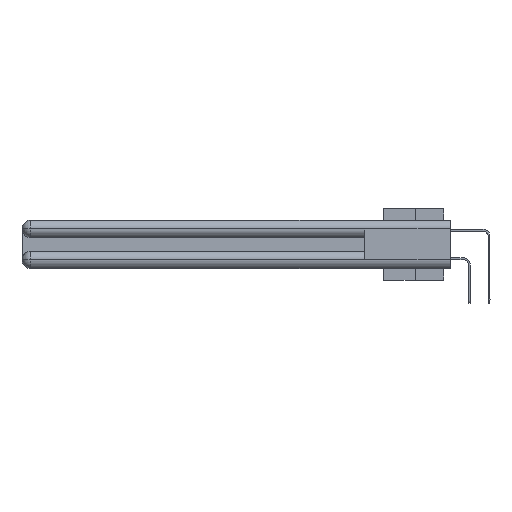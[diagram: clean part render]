
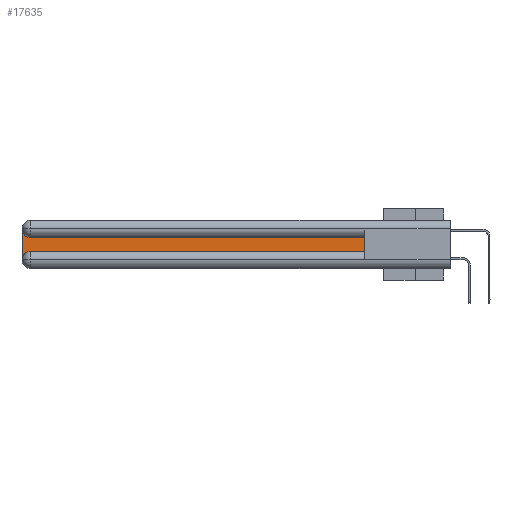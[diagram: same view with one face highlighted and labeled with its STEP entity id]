
A CAD part, left-side view. The second image highlights one B-rep face of the part: STEP entity #17635.
In plain terms, the highlighted planar face has unit normal (-1, 0, 0).
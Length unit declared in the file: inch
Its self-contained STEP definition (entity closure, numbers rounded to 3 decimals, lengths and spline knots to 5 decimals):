
#868 = VERTEX_POINT ( 'NONE', #5775 ) ;
#2789 = VECTOR ( 'NONE', #22124, 39.37008 ) ;
#3018 = VERTEX_POINT ( 'NONE', #8753 ) ;
#3198 = DIRECTION ( 'NONE',  ( 0., 1., 0. ) ) ;
#4186 = CIRCLE ( 'NONE', #22848, 0.06 ) ;
#4320 = ORIENTED_EDGE ( 'NONE', *, *, #15052, .T. ) ;
#4448 = LINE ( 'NONE', #9277, #2789 ) ;
#4522 = LINE ( 'NONE', #17173, #10334 ) ;
#5775 = CARTESIAN_POINT ( 'NONE',  ( 0.075, 2.94, -0.2175 ) ) ;
#5778 = DIRECTION ( 'NONE',  ( 0., 0., -1. ) ) ;
#5838 = CARTESIAN_POINT ( 'NONE',  ( 0.075, 2.94, -0.1225 ) ) ;
#8171 = VERTEX_POINT ( 'NONE', #5838 ) ;
#8753 = CARTESIAN_POINT ( 'NONE',  ( 0.075, 3., -0.2775 ) ) ;
#8764 = CARTESIAN_POINT ( 'NONE',  ( 0.075, 2.94, -0.0625 ) ) ;
#9035 = LINE ( 'NONE', #29760, #17980 ) ;
#9191 = DIRECTION ( 'NONE',  ( 0., -1., 0. ) ) ;
#9277 = CARTESIAN_POINT ( 'NONE',  ( 0.075, 0.6, -0.2175 ) ) ;
#9464 = VECTOR ( 'NONE', #3198, 39.37008 ) ;
#9734 = DIRECTION ( 'NONE',  ( 0., 0., -1. ) ) ;
#10334 = VECTOR ( 'NONE', #19718, 39.37008 ) ;
#12336 = AXIS2_PLACEMENT_3D ( 'NONE', #16892, #27433, #27101 ) ;
#12488 = CARTESIAN_POINT ( 'NONE',  ( 0.075, 3., -0.0625 ) ) ;
#12518 = VERTEX_POINT ( 'NONE', #12488 ) ;
#13029 = EDGE_CURVE ( 'NONE', #8171, #12518, #4186, .T. ) ;
#13334 = CARTESIAN_POINT ( 'NONE',  ( 0.075, 0.6, -0.1225 ) ) ;
#14201 = FACE_OUTER_BOUND ( 'NONE', #30959, .T. ) ;
#15052 = EDGE_CURVE ( 'NONE', #3018, #868, #32667, .T. ) ;
#16786 = ORIENTED_EDGE ( 'NONE', *, *, #17166, .T. ) ;
#16892 = CARTESIAN_POINT ( 'NONE',  ( 0.075, 2.94, -0.2775 ) ) ;
#17166 = EDGE_CURVE ( 'NONE', #23172, #21938, #4448, .T. ) ;
#17173 = CARTESIAN_POINT ( 'NONE',  ( 0.075, 3., -0.2175 ) ) ;
#17635 = ADVANCED_FACE ( 'NONE', ( #14201 ), #24601, .F. ) ;
#17674 = CARTESIAN_POINT ( 'NONE',  ( 0.075, 0.6, -0.1225 ) ) ;
#17980 = VECTOR ( 'NONE', #9191, 39.37008 ) ;
#18822 = AXIS2_PLACEMENT_3D ( 'NONE', #32484, #32653, #9734 ) ;
#18969 = DIRECTION ( 'NONE',  ( 1., 0., 0. ) ) ;
#19718 = DIRECTION ( 'NONE',  ( 0., 0., -1. ) ) ;
#20743 = LINE ( 'NONE', #13334, #9464 ) ;
#21808 = ORIENTED_EDGE ( 'NONE', *, *, #27643, .T. ) ;
#21938 = VERTEX_POINT ( 'NONE', #17674 ) ;
#22124 = DIRECTION ( 'NONE',  ( 0., 0., 1. ) ) ;
#22848 = AXIS2_PLACEMENT_3D ( 'NONE', #8764, #18969, #5778 ) ;
#22881 = ORIENTED_EDGE ( 'NONE', *, *, #23582, .T. ) ;
#23172 = VERTEX_POINT ( 'NONE', #26790 ) ;
#23582 = EDGE_CURVE ( 'NONE', #21938, #8171, #20743, .T. ) ;
#24601 = PLANE ( 'NONE',  #18822 ) ;
#25442 = ORIENTED_EDGE ( 'NONE', *, *, #31390, .T. ) ;
#26790 = CARTESIAN_POINT ( 'NONE',  ( 0.075, 0.6, -0.2175 ) ) ;
#27101 = DIRECTION ( 'NONE',  ( 0., 0., -1. ) ) ;
#27433 = DIRECTION ( 'NONE',  ( 1., 0., 0. ) ) ;
#27643 = EDGE_CURVE ( 'NONE', #12518, #3018, #4522, .T. ) ;
#28111 = ORIENTED_EDGE ( 'NONE', *, *, #13029, .T. ) ;
#29760 = CARTESIAN_POINT ( 'NONE',  ( 0.075, 0.6, -0.2175 ) ) ;
#30959 = EDGE_LOOP ( 'NONE', ( #22881, #28111, #21808, #4320, #25442, #16786 ) ) ;
#31390 = EDGE_CURVE ( 'NONE', #868, #23172, #9035, .T. ) ;
#32484 = CARTESIAN_POINT ( 'NONE',  ( 0.075, 3., -0.1225 ) ) ;
#32653 = DIRECTION ( 'NONE',  ( 1., 0., 0. ) ) ;
#32667 = CIRCLE ( 'NONE', #12336, 0.06 ) ;
